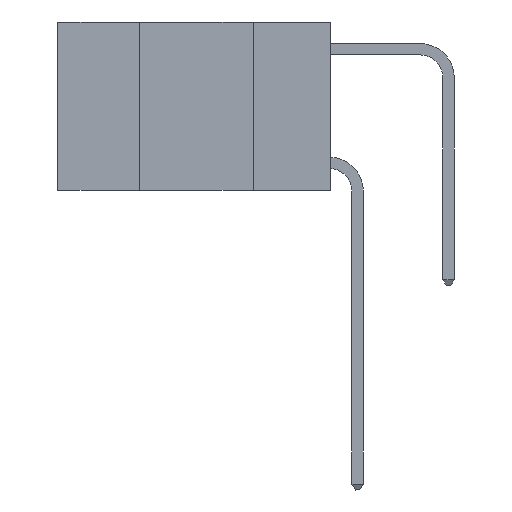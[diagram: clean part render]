
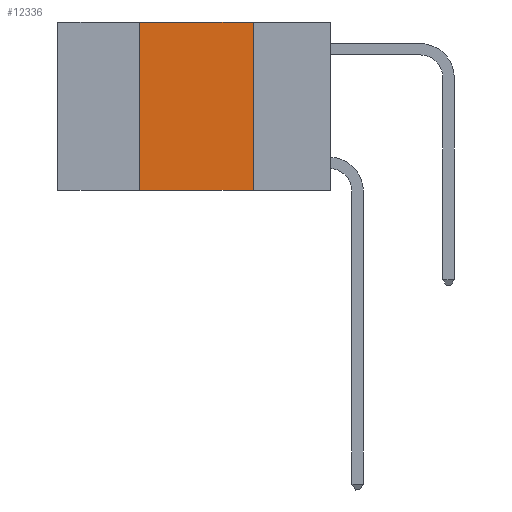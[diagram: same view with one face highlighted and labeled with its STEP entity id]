
A CAD part, left-side view. The second image highlights one B-rep face of the part: STEP entity #12336.
In plain terms, the highlighted planar face has unit normal (-1, 0, 0).
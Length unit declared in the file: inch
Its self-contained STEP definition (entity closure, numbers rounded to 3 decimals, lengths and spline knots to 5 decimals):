
#281 = VECTOR ( 'NONE', #1562, 39.37008 ) ;
#904 = LINE ( 'NONE', #7203, #9766 ) ;
#1562 = DIRECTION ( 'NONE',  ( 0., -1., 0. ) ) ;
#2406 = ORIENTED_EDGE ( 'NONE', *, *, #3404, .F. ) ;
#2955 = EDGE_LOOP ( 'NONE', ( #7061, #3702, #2406, #17034 ) ) ;
#3010 = AXIS2_PLACEMENT_3D ( 'NONE', #19172, #5853, #5636 ) ;
#3091 = EDGE_CURVE ( 'NONE', #9910, #17115, #4431, .T. ) ;
#3404 = EDGE_CURVE ( 'NONE', #9910, #5958, #12261, .T. ) ;
#3702 = ORIENTED_EDGE ( 'NONE', *, *, #16345, .F. ) ;
#4431 = LINE ( 'NONE', #11475, #281 ) ;
#5636 = DIRECTION ( 'NONE',  ( 0., 0., -1. ) ) ;
#5853 = DIRECTION ( 'NONE',  ( 1., 0., 0. ) ) ;
#5955 = CARTESIAN_POINT ( 'NONE',  ( 0., 0.17, 0. ) ) ;
#5958 = VERTEX_POINT ( 'NONE', #8434 ) ;
#7061 = ORIENTED_EDGE ( 'NONE', *, *, #11256, .F. ) ;
#7203 = CARTESIAN_POINT ( 'NONE',  ( 0., 0.6, 0. ) ) ;
#7728 = FACE_OUTER_BOUND ( 'NONE', #2955, .T. ) ;
#8434 = CARTESIAN_POINT ( 'NONE',  ( 0., 0.42, 0. ) ) ;
#9251 = DIRECTION ( 'NONE',  ( 0., 0., 1. ) ) ;
#9570 = CARTESIAN_POINT ( 'NONE',  ( 0., 0.17, -0.37 ) ) ;
#9766 = VECTOR ( 'NONE', #19081, 39.37008 ) ;
#9910 = VERTEX_POINT ( 'NONE', #13536 ) ;
#11007 = CARTESIAN_POINT ( 'NONE',  ( 0., 0.42, 0. ) ) ;
#11256 = EDGE_CURVE ( 'NONE', #15479, #17115, #14885, .T. ) ;
#11475 = CARTESIAN_POINT ( 'NONE',  ( 0., 0.6, -0.37 ) ) ;
#12261 = LINE ( 'NONE', #11007, #19103 ) ;
#12336 = ADVANCED_FACE ( 'NONE', ( #7728 ), #20930, .F. ) ;
#13536 = CARTESIAN_POINT ( 'NONE',  ( 0., 0.42, -0.37 ) ) ;
#14568 = CARTESIAN_POINT ( 'NONE',  ( 0., 0.17, 0. ) ) ;
#14885 = LINE ( 'NONE', #14568, #19143 ) ;
#15479 = VERTEX_POINT ( 'NONE', #5955 ) ;
#16345 = EDGE_CURVE ( 'NONE', #5958, #15479, #904, .T. ) ;
#17034 = ORIENTED_EDGE ( 'NONE', *, *, #3091, .T. ) ;
#17115 = VERTEX_POINT ( 'NONE', #9570 ) ;
#19081 = DIRECTION ( 'NONE',  ( 0., -1., 0. ) ) ;
#19103 = VECTOR ( 'NONE', #9251, 39.37008 ) ;
#19143 = VECTOR ( 'NONE', #21574, 39.37008 ) ;
#19172 = CARTESIAN_POINT ( 'NONE',  ( 0., 0.6, 0. ) ) ;
#20930 = PLANE ( 'NONE',  #3010 ) ;
#21574 = DIRECTION ( 'NONE',  ( 0., 0., -1. ) ) ;
